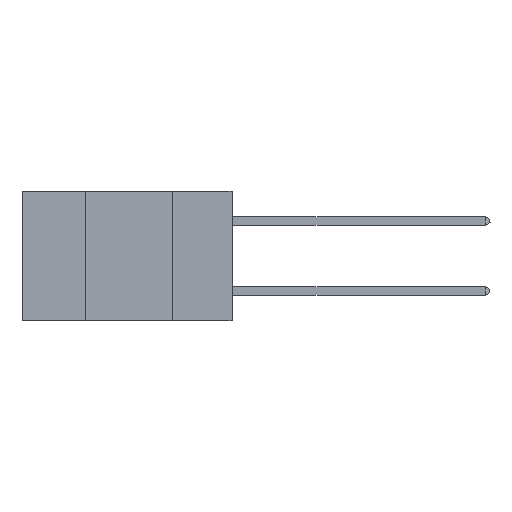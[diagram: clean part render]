
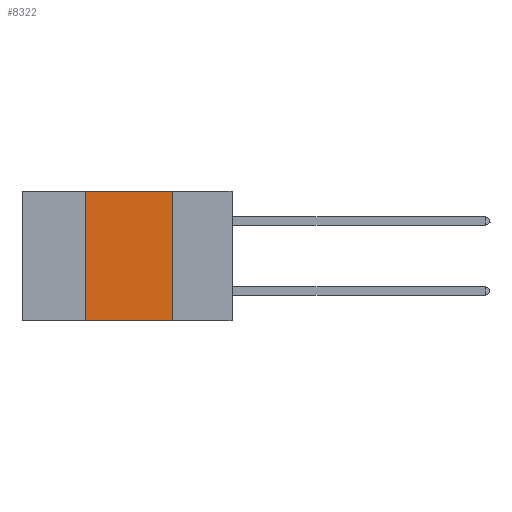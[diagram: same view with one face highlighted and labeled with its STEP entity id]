
A CAD part, left-side view. The second image highlights one B-rep face of the part: STEP entity #8322.
In plain terms, the highlighted planar face has unit normal (-1, 0, 0).
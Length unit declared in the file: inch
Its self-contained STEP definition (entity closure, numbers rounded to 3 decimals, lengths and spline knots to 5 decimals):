
#1093 = DIRECTION ( 'NONE',  ( 0., 0., -1. ) ) ;
#1397 = VECTOR ( 'NONE', #1890, 39.37008 ) ;
#1711 = CARTESIAN_POINT ( 'NONE',  ( 0., 0.42, 0. ) ) ;
#1890 = DIRECTION ( 'NONE',  ( 0., -1., 0. ) ) ;
#2121 = CARTESIAN_POINT ( 'NONE',  ( 0., 0.6, 0. ) ) ;
#2130 = CARTESIAN_POINT ( 'NONE',  ( 0., 0.17, -0.37 ) ) ;
#2417 = VECTOR ( 'NONE', #12035, 39.37008 ) ;
#3779 = VECTOR ( 'NONE', #5156, 39.37008 ) ;
#3850 = CARTESIAN_POINT ( 'NONE',  ( 0., 0.42, -0.37 ) ) ;
#3888 = CARTESIAN_POINT ( 'NONE',  ( 0., 0.17, 0. ) ) ;
#4460 = VERTEX_POINT ( 'NONE', #3850 ) ;
#4469 = ORIENTED_EDGE ( 'NONE', *, *, #9871, .F. ) ;
#5156 = DIRECTION ( 'NONE',  ( 0., 0., 1. ) ) ;
#5171 = DIRECTION ( 'NONE',  ( 0., 0., -1. ) ) ;
#5228 = LINE ( 'NONE', #12050, #1397 ) ;
#5243 = DIRECTION ( 'NONE',  ( 1., 0., 0. ) ) ;
#5627 = CARTESIAN_POINT ( 'NONE',  ( 0., 0.17, 0. ) ) ;
#6318 = ORIENTED_EDGE ( 'NONE', *, *, #10018, .T. ) ;
#7455 = ORIENTED_EDGE ( 'NONE', *, *, #12366, .F. ) ;
#7742 = FACE_OUTER_BOUND ( 'NONE', #13896, .T. ) ;
#7782 = VERTEX_POINT ( 'NONE', #3888 ) ;
#8063 = CARTESIAN_POINT ( 'NONE',  ( 0., 0.42, 0. ) ) ;
#8322 = ADVANCED_FACE ( 'NONE', ( #7742 ), #11176, .F. ) ;
#8620 = LINE ( 'NONE', #13312, #2417 ) ;
#9536 = LINE ( 'NONE', #8063, #3779 ) ;
#9594 = VERTEX_POINT ( 'NONE', #1711 ) ;
#9860 = AXIS2_PLACEMENT_3D ( 'NONE', #2121, #5243, #5171 ) ;
#9871 = EDGE_CURVE ( 'NONE', #4460, #9594, #9536, .T. ) ;
#10018 = EDGE_CURVE ( 'NONE', #4460, #14004, #5228, .T. ) ;
#10217 = LINE ( 'NONE', #5627, #14498 ) ;
#11176 = PLANE ( 'NONE',  #9860 ) ;
#12035 = DIRECTION ( 'NONE',  ( 0., -1., 0. ) ) ;
#12050 = CARTESIAN_POINT ( 'NONE',  ( 0., 0.6, -0.37 ) ) ;
#12366 = EDGE_CURVE ( 'NONE', #7782, #14004, #10217, .T. ) ;
#13312 = CARTESIAN_POINT ( 'NONE',  ( 0., 0.6, 0. ) ) ;
#13369 = ORIENTED_EDGE ( 'NONE', *, *, #13595, .F. ) ;
#13595 = EDGE_CURVE ( 'NONE', #9594, #7782, #8620, .T. ) ;
#13896 = EDGE_LOOP ( 'NONE', ( #7455, #13369, #4469, #6318 ) ) ;
#14004 = VERTEX_POINT ( 'NONE', #2130 ) ;
#14498 = VECTOR ( 'NONE', #1093, 39.37008 ) ;
